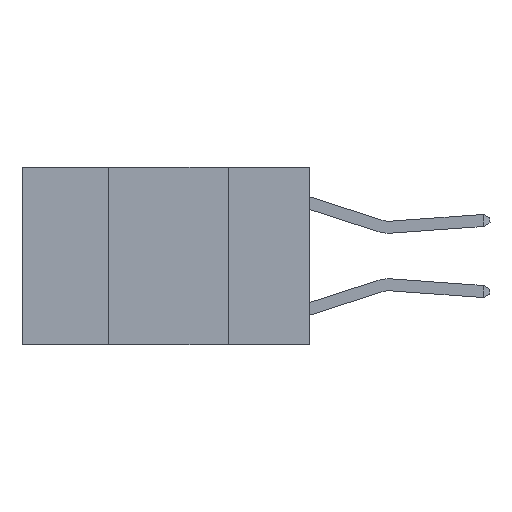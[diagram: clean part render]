
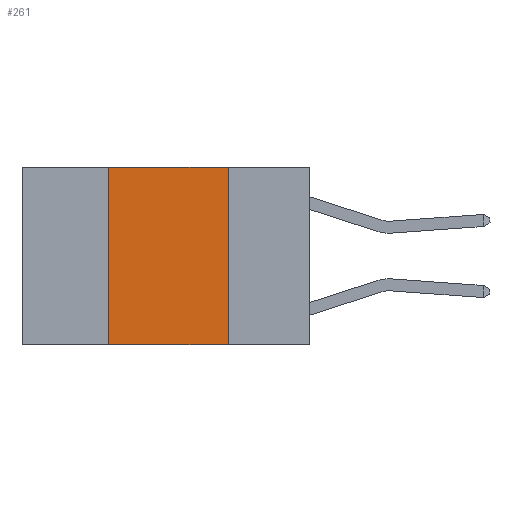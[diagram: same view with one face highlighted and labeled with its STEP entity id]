
A CAD part, left-side view. The second image highlights one B-rep face of the part: STEP entity #261.
In plain terms, the highlighted planar face has unit normal (-1, 0, 0).
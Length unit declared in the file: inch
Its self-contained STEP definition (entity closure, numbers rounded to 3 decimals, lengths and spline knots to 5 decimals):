
#261 = ADVANCED_FACE ( 'NONE', ( #8998 ), #6308, .F. ) ;
#471 = DIRECTION ( 'NONE',  ( 0., 0., -1. ) ) ;
#592 = ORIENTED_EDGE ( 'NONE', *, *, #12672, .T. ) ;
#1548 = CARTESIAN_POINT ( 'NONE',  ( 0., 0.17, 0. ) ) ;
#2250 = VERTEX_POINT ( 'NONE', #9685 ) ;
#2485 = LINE ( 'NONE', #10500, #16624 ) ;
#2714 = EDGE_CURVE ( 'NONE', #2250, #3203, #3560, .T. ) ;
#3203 = VERTEX_POINT ( 'NONE', #1548 ) ;
#3560 = LINE ( 'NONE', #9167, #14420 ) ;
#3623 = ORIENTED_EDGE ( 'NONE', *, *, #2714, .F. ) ;
#3631 = VECTOR ( 'NONE', #15768, 39.37008 ) ;
#3731 = EDGE_LOOP ( 'NONE', ( #14478, #3623, #15356, #592 ) ) ;
#4354 = CARTESIAN_POINT ( 'NONE',  ( 0., 0.42, -0.37 ) ) ;
#4984 = DIRECTION ( 'NONE',  ( 0., -1., 0. ) ) ;
#4996 = DIRECTION ( 'NONE',  ( 0., 0., -1. ) ) ;
#5111 = VECTOR ( 'NONE', #17609, 39.37008 ) ;
#5427 = DIRECTION ( 'NONE',  ( 1., 0., 0. ) ) ;
#5812 = CARTESIAN_POINT ( 'NONE',  ( 0., 0.17, -0.37 ) ) ;
#5908 = CARTESIAN_POINT ( 'NONE',  ( 0., 0.42, 0. ) ) ;
#6308 = PLANE ( 'NONE',  #16344 ) ;
#6455 = CARTESIAN_POINT ( 'NONE',  ( 0., 0.6, -0.37 ) ) ;
#7645 = EDGE_CURVE ( 'NONE', #3203, #16515, #2485, .T. ) ;
#8998 = FACE_OUTER_BOUND ( 'NONE', #3731, .T. ) ;
#9167 = CARTESIAN_POINT ( 'NONE',  ( 0., 0.6, 0. ) ) ;
#9685 = CARTESIAN_POINT ( 'NONE',  ( 0., 0.42, 0. ) ) ;
#10364 = VERTEX_POINT ( 'NONE', #4354 ) ;
#10500 = CARTESIAN_POINT ( 'NONE',  ( 0., 0.17, 0. ) ) ;
#12672 = EDGE_CURVE ( 'NONE', #10364, #16515, #14374, .T. ) ;
#14374 = LINE ( 'NONE', #6455, #5111 ) ;
#14420 = VECTOR ( 'NONE', #4984, 39.37008 ) ;
#14478 = ORIENTED_EDGE ( 'NONE', *, *, #7645, .F. ) ;
#14497 = LINE ( 'NONE', #5908, #3631 ) ;
#14882 = CARTESIAN_POINT ( 'NONE',  ( 0., 0.6, 0. ) ) ;
#15356 = ORIENTED_EDGE ( 'NONE', *, *, #17313, .F. ) ;
#15768 = DIRECTION ( 'NONE',  ( 0., 0., 1. ) ) ;
#16344 = AXIS2_PLACEMENT_3D ( 'NONE', #14882, #5427, #4996 ) ;
#16515 = VERTEX_POINT ( 'NONE', #5812 ) ;
#16624 = VECTOR ( 'NONE', #471, 39.37008 ) ;
#17313 = EDGE_CURVE ( 'NONE', #10364, #2250, #14497, .T. ) ;
#17609 = DIRECTION ( 'NONE',  ( 0., -1., 0. ) ) ;
